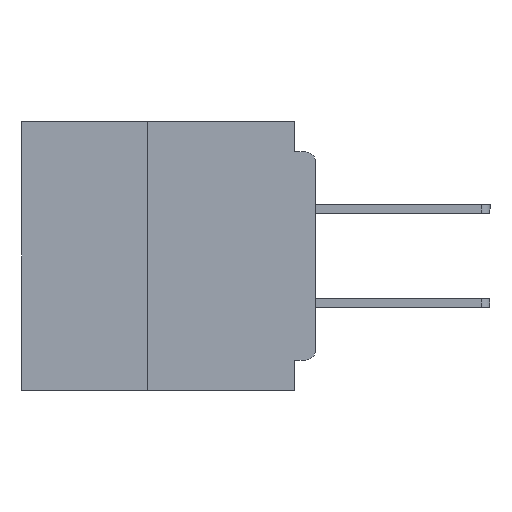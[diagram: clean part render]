
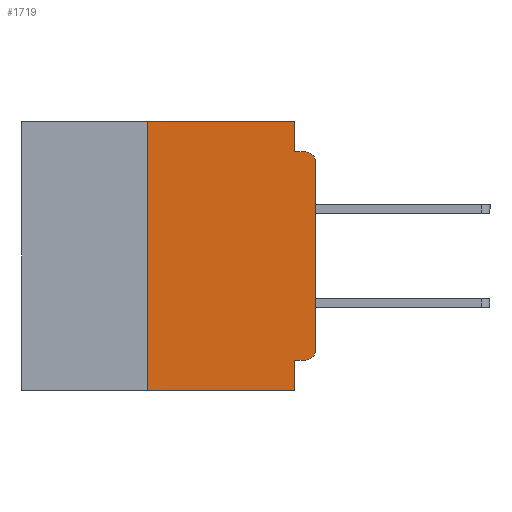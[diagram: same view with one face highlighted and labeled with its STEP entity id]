
A CAD part, left-side view. The second image highlights one B-rep face of the part: STEP entity #1719.
In plain terms, the highlighted planar face has unit normal (-1, 0, 0).
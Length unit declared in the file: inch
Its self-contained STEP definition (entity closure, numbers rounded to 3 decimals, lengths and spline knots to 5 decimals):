
#256 = DIRECTION ( 'NONE',  ( 0., -1., 0. ) ) ;
#1339 = ORIENTED_EDGE ( 'NONE', *, *, #2463, .F. ) ;
#1719 = ADVANCED_FACE ( 'NONE', ( #15224 ), #28625, .F. ) ;
#1815 = VECTOR ( 'NONE', #15986, 39.37008 ) ;
#2025 = CARTESIAN_POINT ( 'NONE',  ( 0., 0.015, -0.045 ) ) ;
#2463 = EDGE_CURVE ( 'NONE', #9292, #8936, #27558, .T. ) ;
#2984 = VECTOR ( 'NONE', #20680, 39.37008 ) ;
#3662 = ORIENTED_EDGE ( 'NONE', *, *, #23005, .F. ) ;
#4230 = ORIENTED_EDGE ( 'NONE', *, *, #23395, .F. ) ;
#5050 = LINE ( 'NONE', #15051, #11262 ) ;
#6568 = ORIENTED_EDGE ( 'NONE', *, *, #18623, .T. ) ;
#6983 = VERTEX_POINT ( 'NONE', #9040 ) ;
#7664 = VECTOR ( 'NONE', #23168, 39.37008 ) ;
#8199 = EDGE_CURVE ( 'NONE', #44827, #17095, #39094, .T. ) ;
#8617 = CARTESIAN_POINT ( 'NONE',  ( 0., 0., -0.045 ) ) ;
#8700 = ORIENTED_EDGE ( 'NONE', *, *, #19444, .F. ) ;
#8757 = CARTESIAN_POINT ( 'NONE',  ( 0., 0., 0. ) ) ;
#8936 = VERTEX_POINT ( 'NONE', #41999 ) ;
#9040 = CARTESIAN_POINT ( 'NONE',  ( 0., 0., -0.06 ) ) ;
#9292 = VERTEX_POINT ( 'NONE', #26080 ) ;
#10916 = ORIENTED_EDGE ( 'NONE', *, *, #17357, .T. ) ;
#11262 = VECTOR ( 'NONE', #36621, 39.37008 ) ;
#12030 = EDGE_CURVE ( 'NONE', #20591, #6983, #36512, .T. ) ;
#12756 = CARTESIAN_POINT ( 'NONE',  ( 0., 0.437, 0. ) ) ;
#12818 = CARTESIAN_POINT ( 'NONE',  ( 0., 0.031, -0.4 ) ) ;
#13144 = VERTEX_POINT ( 'NONE', #29512 ) ;
#13454 = ORIENTED_EDGE ( 'NONE', *, *, #8199, .F. ) ;
#13885 = EDGE_LOOP ( 'NONE', ( #21918, #6568, #13454, #41463, #8700, #1339, #16955, #3662, #4230, #10916 ) ) ;
#14746 = CARTESIAN_POINT ( 'NONE',  ( 0., 0.015, -0.06 ) ) ;
#15051 = CARTESIAN_POINT ( 'NONE',  ( 0., 0., -0.355 ) ) ;
#15224 = FACE_OUTER_BOUND ( 'NONE', #13885, .T. ) ;
#15986 = DIRECTION ( 'NONE',  ( 0., -1., 0. ) ) ;
#16955 = ORIENTED_EDGE ( 'NONE', *, *, #31333, .T. ) ;
#17084 = CARTESIAN_POINT ( 'NONE',  ( 0., 0.031, 0. ) ) ;
#17095 = VERTEX_POINT ( 'NONE', #2025 ) ;
#17357 = EDGE_CURVE ( 'NONE', #13144, #20591, #17424, .T. ) ;
#17424 = CIRCLE ( 'NONE', #24473, 0.015 ) ;
#17854 = CARTESIAN_POINT ( 'NONE',  ( 0., 0.015, -0.34 ) ) ;
#18005 = VECTOR ( 'NONE', #18165, 39.37008 ) ;
#18165 = DIRECTION ( 'NONE',  ( 0., 0., 1. ) ) ;
#18360 = DIRECTION ( 'NONE',  ( 0., 0., -1. ) ) ;
#18397 = CIRCLE ( 'NONE', #24813, 0.015 ) ;
#18623 = EDGE_CURVE ( 'NONE', #6983, #17095, #18397, .T. ) ;
#19442 = CARTESIAN_POINT ( 'NONE',  ( 0., 0.031, -0.045 ) ) ;
#19444 = EDGE_CURVE ( 'NONE', #8936, #35247, #23942, .T. ) ;
#20340 = CARTESIAN_POINT ( 'NONE',  ( 0., 0.031, -0.4 ) ) ;
#20509 = VERTEX_POINT ( 'NONE', #20340 ) ;
#20591 = VERTEX_POINT ( 'NONE', #38616 ) ;
#20680 = DIRECTION ( 'NONE',  ( 0., 0., -1. ) ) ;
#21465 = DIRECTION ( 'NONE',  ( 0., 0., -1. ) ) ;
#21918 = ORIENTED_EDGE ( 'NONE', *, *, #12030, .T. ) ;
#21936 = CARTESIAN_POINT ( 'NONE',  ( 0., 0.437, -0.4 ) ) ;
#23005 = EDGE_CURVE ( 'NONE', #41273, #20509, #24227, .T. ) ;
#23168 = DIRECTION ( 'NONE',  ( 0., 0., 1. ) ) ;
#23395 = EDGE_CURVE ( 'NONE', #13144, #41273, #5050, .T. ) ;
#23460 = AXIS2_PLACEMENT_3D ( 'NONE', #28591, #28474, #28337 ) ;
#23713 = CARTESIAN_POINT ( 'NONE',  ( 0., 0.031, 0. ) ) ;
#23942 = LINE ( 'NONE', #12756, #30130 ) ;
#24227 = LINE ( 'NONE', #12818, #32727 ) ;
#24473 = AXIS2_PLACEMENT_3D ( 'NONE', #17854, #42955, #21465 ) ;
#24813 = AXIS2_PLACEMENT_3D ( 'NONE', #14746, #39917, #18360 ) ;
#26080 = CARTESIAN_POINT ( 'NONE',  ( 0., 0.25, -0.4 ) ) ;
#27558 = LINE ( 'NONE', #39717, #18005 ) ;
#28337 = DIRECTION ( 'NONE',  ( 0., 0., -1. ) ) ;
#28474 = DIRECTION ( 'NONE',  ( 1., 0., 0. ) ) ;
#28591 = CARTESIAN_POINT ( 'NONE',  ( 0., 0.437, 0. ) ) ;
#28625 = PLANE ( 'NONE',  #23460 ) ;
#29512 = CARTESIAN_POINT ( 'NONE',  ( 0., 0.015, -0.355 ) ) ;
#30130 = VECTOR ( 'NONE', #38010, 39.37008 ) ;
#30803 = DIRECTION ( 'NONE',  ( 0., 0., -1. ) ) ;
#31333 = EDGE_CURVE ( 'NONE', #9292, #20509, #42850, .T. ) ;
#32727 = VECTOR ( 'NONE', #30803, 39.37008 ) ;
#33344 = CARTESIAN_POINT ( 'NONE',  ( 0., 0.031, -0.355 ) ) ;
#33395 = VECTOR ( 'NONE', #256, 39.37008 ) ;
#35247 = VERTEX_POINT ( 'NONE', #23713 ) ;
#35941 = EDGE_CURVE ( 'NONE', #35247, #44827, #41392, .T. ) ;
#36512 = LINE ( 'NONE', #8757, #7664 ) ;
#36621 = DIRECTION ( 'NONE',  ( 0., 1., 0. ) ) ;
#38010 = DIRECTION ( 'NONE',  ( 0., -1., 0. ) ) ;
#38616 = CARTESIAN_POINT ( 'NONE',  ( 0., 0., -0.34 ) ) ;
#39094 = LINE ( 'NONE', #8617, #1815 ) ;
#39717 = CARTESIAN_POINT ( 'NONE',  ( 0., 0.25, -0.4 ) ) ;
#39917 = DIRECTION ( 'NONE',  ( -1., 0., 0. ) ) ;
#41273 = VERTEX_POINT ( 'NONE', #33344 ) ;
#41392 = LINE ( 'NONE', #17084, #2984 ) ;
#41463 = ORIENTED_EDGE ( 'NONE', *, *, #35941, .F. ) ;
#41999 = CARTESIAN_POINT ( 'NONE',  ( 0., 0.25, 0. ) ) ;
#42850 = LINE ( 'NONE', #21936, #33395 ) ;
#42955 = DIRECTION ( 'NONE',  ( -1., 0., 0. ) ) ;
#44827 = VERTEX_POINT ( 'NONE', #19442 ) ;
